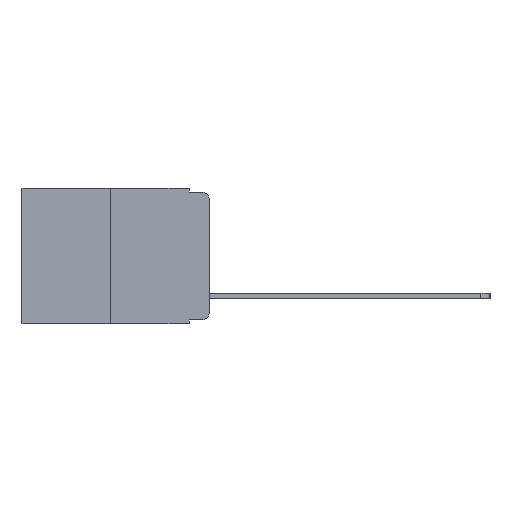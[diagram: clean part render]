
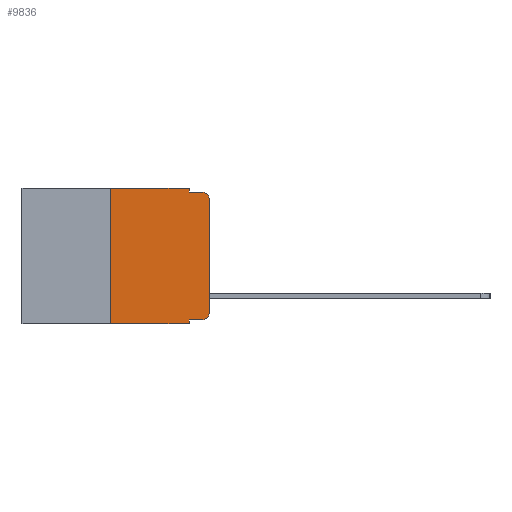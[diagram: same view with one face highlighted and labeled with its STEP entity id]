
A CAD part, left-side view. The second image highlights one B-rep face of the part: STEP entity #9836.
In plain terms, the highlighted planar face has unit normal (-1, 0, 0).
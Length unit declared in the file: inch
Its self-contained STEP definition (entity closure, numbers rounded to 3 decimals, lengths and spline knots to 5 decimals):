
#6 = LINE ( 'NONE', #12204, #3359 ) ;
#358 = CARTESIAN_POINT ( 'NONE',  ( 0., 0.25, -0.343 ) ) ;
#401 = EDGE_CURVE ( 'NONE', #2524, #14068, #7106, .T. ) ;
#509 = CARTESIAN_POINT ( 'NONE',  ( 0., 0.02, -0.01 ) ) ;
#878 = ORIENTED_EDGE ( 'NONE', *, *, #5653, .T. ) ;
#1308 = EDGE_CURVE ( 'NONE', #2711, #6376, #6, .T. ) ;
#1343 = VERTEX_POINT ( 'NONE', #4892 ) ;
#1481 = CARTESIAN_POINT ( 'NONE',  ( 0., 0.051, -0.333 ) ) ;
#1792 = VERTEX_POINT ( 'NONE', #11003 ) ;
#1807 = CARTESIAN_POINT ( 'NONE',  ( 0., 0.02, -0.313 ) ) ;
#2461 = DIRECTION ( 'NONE',  ( 0., -1., 0. ) ) ;
#2485 = VECTOR ( 'NONE', #10072, 39.37008 ) ;
#2524 = VERTEX_POINT ( 'NONE', #358 ) ;
#2532 = AXIS2_PLACEMENT_3D ( 'NONE', #1807, #9492, #2929 ) ;
#2634 = CARTESIAN_POINT ( 'NONE',  ( 0., 0., -0.03 ) ) ;
#2711 = VERTEX_POINT ( 'NONE', #11193 ) ;
#2929 = DIRECTION ( 'NONE',  ( 0., 0., -1. ) ) ;
#3035 = LINE ( 'NONE', #13631, #11329 ) ;
#3139 = ORIENTED_EDGE ( 'NONE', *, *, #7890, .T. ) ;
#3359 = VECTOR ( 'NONE', #4433, 39.37008 ) ;
#3689 = CARTESIAN_POINT ( 'NONE',  ( 0., 0.473, 0. ) ) ;
#4248 = ORIENTED_EDGE ( 'NONE', *, *, #11500, .T. ) ;
#4257 = LINE ( 'NONE', #1481, #6881 ) ;
#4357 = VECTOR ( 'NONE', #4932, 39.37008 ) ;
#4374 = ORIENTED_EDGE ( 'NONE', *, *, #4989, .F. ) ;
#4433 = DIRECTION ( 'NONE',  ( 0., 0., -1. ) ) ;
#4617 = CIRCLE ( 'NONE', #6763, 0.02 ) ;
#4649 = CARTESIAN_POINT ( 'NONE',  ( 0., 0.051, 0. ) ) ;
#4776 = CARTESIAN_POINT ( 'NONE',  ( 0., 0.25, 0. ) ) ;
#4892 = CARTESIAN_POINT ( 'NONE',  ( 0., 0.051, 0. ) ) ;
#4932 = DIRECTION ( 'NONE',  ( 0., -1., 0. ) ) ;
#4989 = EDGE_CURVE ( 'NONE', #7976, #12352, #9245, .T. ) ;
#5204 = CARTESIAN_POINT ( 'NONE',  ( 0., 0.02, -0.03 ) ) ;
#5350 = LINE ( 'NONE', #7974, #11379 ) ;
#5653 = EDGE_CURVE ( 'NONE', #2711, #13068, #4257, .T. ) ;
#5932 = DIRECTION ( 'NONE',  ( 0., 0., -1. ) ) ;
#6344 = DIRECTION ( 'NONE',  ( 0., 0., -1. ) ) ;
#6376 = VERTEX_POINT ( 'NONE', #12181 ) ;
#6392 = VECTOR ( 'NONE', #12029, 39.37008 ) ;
#6763 = AXIS2_PLACEMENT_3D ( 'NONE', #5204, #12713, #6344 ) ;
#6881 = VECTOR ( 'NONE', #2461, 39.37008 ) ;
#7106 = LINE ( 'NONE', #11470, #10902 ) ;
#7164 = EDGE_CURVE ( 'NONE', #14068, #1343, #8031, .T. ) ;
#7333 = AXIS2_PLACEMENT_3D ( 'NONE', #3689, #12322, #5932 ) ;
#7737 = ORIENTED_EDGE ( 'NONE', *, *, #7164, .F. ) ;
#7890 = EDGE_CURVE ( 'NONE', #13068, #1792, #10487, .T. ) ;
#7949 = DIRECTION ( 'NONE',  ( 0., -1., 0. ) ) ;
#7974 = CARTESIAN_POINT ( 'NONE',  ( 0., 0., 0. ) ) ;
#7976 = VERTEX_POINT ( 'NONE', #9585 ) ;
#8031 = LINE ( 'NONE', #12455, #4357 ) ;
#8941 = FACE_OUTER_BOUND ( 'NONE', #12827, .T. ) ;
#9245 = LINE ( 'NONE', #12413, #6392 ) ;
#9270 = VERTEX_POINT ( 'NONE', #2634 ) ;
#9492 = DIRECTION ( 'NONE',  ( -1., 0., 0. ) ) ;
#9585 = CARTESIAN_POINT ( 'NONE',  ( 0., 0.051, -0.01 ) ) ;
#9687 = ORIENTED_EDGE ( 'NONE', *, *, #12179, .F. ) ;
#9836 = ADVANCED_FACE ( 'NONE', ( #8941 ), #10194, .F. ) ;
#10072 = DIRECTION ( 'NONE',  ( 0., 0., -1. ) ) ;
#10194 = PLANE ( 'NONE',  #7333 ) ;
#10340 = EDGE_CURVE ( 'NONE', #9270, #12352, #4617, .T. ) ;
#10460 = CARTESIAN_POINT ( 'NONE',  ( 0., 0.02, -0.333 ) ) ;
#10487 = CIRCLE ( 'NONE', #2532, 0.02 ) ;
#10825 = LINE ( 'NONE', #4649, #2485 ) ;
#10902 = VECTOR ( 'NONE', #11058, 39.37008 ) ;
#10996 = ORIENTED_EDGE ( 'NONE', *, *, #10340, .T. ) ;
#11003 = CARTESIAN_POINT ( 'NONE',  ( 0., 0., -0.313 ) ) ;
#11058 = DIRECTION ( 'NONE',  ( 0., 0., 1. ) ) ;
#11193 = CARTESIAN_POINT ( 'NONE',  ( 0., 0.051, -0.333 ) ) ;
#11329 = VECTOR ( 'NONE', #7949, 39.37008 ) ;
#11379 = VECTOR ( 'NONE', #12131, 39.37008 ) ;
#11470 = CARTESIAN_POINT ( 'NONE',  ( 0., 0.25, 0. ) ) ;
#11500 = EDGE_CURVE ( 'NONE', #2524, #6376, #3035, .T. ) ;
#11908 = ORIENTED_EDGE ( 'NONE', *, *, #1308, .F. ) ;
#12029 = DIRECTION ( 'NONE',  ( 0., -1., 0. ) ) ;
#12131 = DIRECTION ( 'NONE',  ( 0., 0., 1. ) ) ;
#12179 = EDGE_CURVE ( 'NONE', #1343, #7976, #10825, .T. ) ;
#12181 = CARTESIAN_POINT ( 'NONE',  ( 0., 0.051, -0.343 ) ) ;
#12204 = CARTESIAN_POINT ( 'NONE',  ( 0., 0.051, 0. ) ) ;
#12322 = DIRECTION ( 'NONE',  ( 1., 0., 0. ) ) ;
#12352 = VERTEX_POINT ( 'NONE', #509 ) ;
#12413 = CARTESIAN_POINT ( 'NONE',  ( 0., 0.051, -0.01 ) ) ;
#12455 = CARTESIAN_POINT ( 'NONE',  ( 0., 0.473, 0. ) ) ;
#12636 = ORIENTED_EDGE ( 'NONE', *, *, #401, .F. ) ;
#12713 = DIRECTION ( 'NONE',  ( -1., 0., 0. ) ) ;
#12827 = EDGE_LOOP ( 'NONE', ( #13601, #10996, #4374, #9687, #7737, #12636, #4248, #11908, #878, #3139 ) ) ;
#13068 = VERTEX_POINT ( 'NONE', #10460 ) ;
#13451 = EDGE_CURVE ( 'NONE', #1792, #9270, #5350, .T. ) ;
#13601 = ORIENTED_EDGE ( 'NONE', *, *, #13451, .T. ) ;
#13631 = CARTESIAN_POINT ( 'NONE',  ( 0., 0.473, -0.343 ) ) ;
#14068 = VERTEX_POINT ( 'NONE', #4776 ) ;
